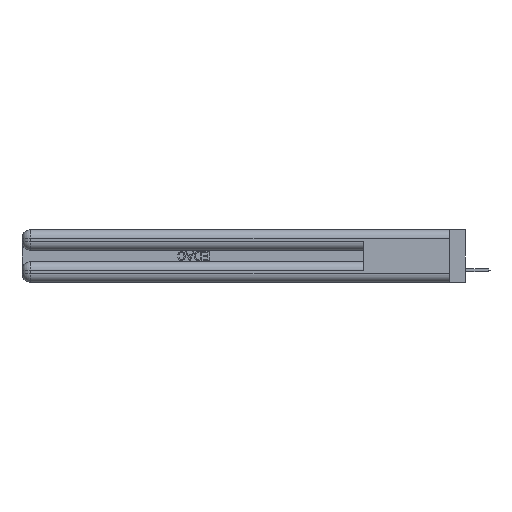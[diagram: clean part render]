
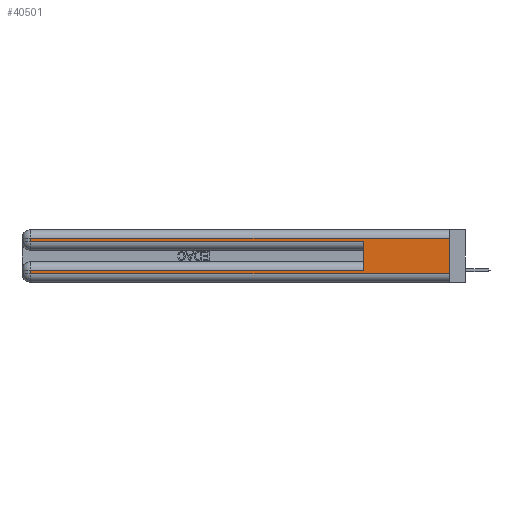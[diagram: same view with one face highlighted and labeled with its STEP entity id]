
A CAD part, left-side view. The second image highlights one B-rep face of the part: STEP entity #40501.
In plain terms, the highlighted planar face has unit normal (-1, 0, 0).
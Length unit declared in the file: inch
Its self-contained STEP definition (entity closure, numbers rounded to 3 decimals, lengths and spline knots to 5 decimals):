
#38 = ORIENTED_EDGE ( 'NONE', *, *, #3209, .T. ) ;
#980 = CARTESIAN_POINT ( 'NONE',  ( 0., 2.94, 0.37 ) ) ;
#3001 = DIRECTION ( 'NONE',  ( 1., 0., 0. ) ) ;
#3209 = EDGE_CURVE ( 'NONE', #36364, #26519, #8917, .T. ) ;
#5085 = VERTEX_POINT ( 'NONE', #32328 ) ;
#5512 = LINE ( 'NONE', #980, #37307 ) ;
#7066 = FACE_OUTER_BOUND ( 'NONE', #13758, .T. ) ;
#8419 = LINE ( 'NONE', #53449, #38146 ) ;
#8917 = LINE ( 'NONE', #11844, #48561 ) ;
#9358 = LINE ( 'NONE', #31911, #36074 ) ;
#9400 = VECTOR ( 'NONE', #47219, 39.37008 ) ;
#9889 = CARTESIAN_POINT ( 'NONE',  ( 0., 2.94, 0.31 ) ) ;
#11844 = CARTESIAN_POINT ( 'NONE',  ( 0., 0., 0.31 ) ) ;
#12064 = EDGE_CURVE ( 'NONE', #26519, #24827, #35401, .T. ) ;
#13758 = EDGE_LOOP ( 'NONE', ( #24534, #38, #50159, #14499, #49826, #46130, #17856, #27384 ) ) ;
#14499 = ORIENTED_EDGE ( 'NONE', *, *, #36199, .T. ) ;
#14515 = LINE ( 'NONE', #39742, #15880 ) ;
#15880 = VECTOR ( 'NONE', #31403, 39.37008 ) ;
#16010 = DIRECTION ( 'NONE',  ( 0., 0., -1. ) ) ;
#17319 = CARTESIAN_POINT ( 'NONE',  ( 0., 0., 0.37 ) ) ;
#17576 = VERTEX_POINT ( 'NONE', #41421 ) ;
#17856 = ORIENTED_EDGE ( 'NONE', *, *, #25757, .T. ) ;
#18302 = CARTESIAN_POINT ( 'NONE',  ( 0., 0., 0.37 ) ) ;
#23362 = EDGE_CURVE ( 'NONE', #23392, #32150, #8419, .T. ) ;
#23392 = VERTEX_POINT ( 'NONE', #47126 ) ;
#23675 = LINE ( 'NONE', #18302, #42400 ) ;
#24534 = ORIENTED_EDGE ( 'NONE', *, *, #44513, .F. ) ;
#24827 = VERTEX_POINT ( 'NONE', #48886 ) ;
#25757 = EDGE_CURVE ( 'NONE', #33454, #17576, #5512, .T. ) ;
#26248 = DIRECTION ( 'NONE',  ( 0., 0., 1. ) ) ;
#26257 = CARTESIAN_POINT ( 'NONE',  ( 0., 2.94, 0.085 ) ) ;
#26311 = DIRECTION ( 'NONE',  ( 0., 0., -1. ) ) ;
#26519 = VERTEX_POINT ( 'NONE', #9889 ) ;
#27384 = ORIENTED_EDGE ( 'NONE', *, *, #44716, .T. ) ;
#28302 = DIRECTION ( 'NONE',  ( 0., 1., 0. ) ) ;
#30276 = DIRECTION ( 'NONE',  ( 0., 0., -1. ) ) ;
#30992 = DIRECTION ( 'NONE',  ( 0., -1., 0. ) ) ;
#31403 = DIRECTION ( 'NONE',  ( 0., -1., 0. ) ) ;
#31911 = CARTESIAN_POINT ( 'NONE',  ( 0., 0., 0.285 ) ) ;
#32150 = VERTEX_POINT ( 'NONE', #51541 ) ;
#32328 = CARTESIAN_POINT ( 'NONE',  ( 0., 0., 0.06 ) ) ;
#33033 = LINE ( 'NONE', #44032, #36967 ) ;
#33454 = VERTEX_POINT ( 'NONE', #26257 ) ;
#35401 = LINE ( 'NONE', #48009, #9400 ) ;
#36074 = VECTOR ( 'NONE', #30992, 39.37008 ) ;
#36199 = EDGE_CURVE ( 'NONE', #24827, #32150, #9358, .T. ) ;
#36364 = VERTEX_POINT ( 'NONE', #39438 ) ;
#36967 = VECTOR ( 'NONE', #28302, 39.37008 ) ;
#37307 = VECTOR ( 'NONE', #26311, 39.37008 ) ;
#38146 = VECTOR ( 'NONE', #26248, 39.37008 ) ;
#39438 = CARTESIAN_POINT ( 'NONE',  ( 0., 0., 0.31 ) ) ;
#39742 = CARTESIAN_POINT ( 'NONE',  ( 0., 0., 0.06 ) ) ;
#40501 = ADVANCED_FACE ( 'NONE', ( #7066 ), #44426, .F. ) ;
#41421 = CARTESIAN_POINT ( 'NONE',  ( 0., 2.94, 0.06 ) ) ;
#42400 = VECTOR ( 'NONE', #30276, 39.37008 ) ;
#44032 = CARTESIAN_POINT ( 'NONE',  ( 0., 0., 0.085 ) ) ;
#44426 = PLANE ( 'NONE',  #45431 ) ;
#44513 = EDGE_CURVE ( 'NONE', #36364, #5085, #23675, .T. ) ;
#44716 = EDGE_CURVE ( 'NONE', #17576, #5085, #14515, .T. ) ;
#45431 = AXIS2_PLACEMENT_3D ( 'NONE', #17319, #3001, #16010 ) ;
#46130 = ORIENTED_EDGE ( 'NONE', *, *, #51348, .T. ) ;
#47126 = CARTESIAN_POINT ( 'NONE',  ( 0., 0.6, 0.085 ) ) ;
#47219 = DIRECTION ( 'NONE',  ( 0., 0., -1. ) ) ;
#48009 = CARTESIAN_POINT ( 'NONE',  ( 0., 2.94, 0.37 ) ) ;
#48561 = VECTOR ( 'NONE', #48981, 39.37008 ) ;
#48886 = CARTESIAN_POINT ( 'NONE',  ( 0., 2.94, 0.285 ) ) ;
#48981 = DIRECTION ( 'NONE',  ( 0., 1., 0. ) ) ;
#49826 = ORIENTED_EDGE ( 'NONE', *, *, #23362, .F. ) ;
#50159 = ORIENTED_EDGE ( 'NONE', *, *, #12064, .T. ) ;
#51348 = EDGE_CURVE ( 'NONE', #23392, #33454, #33033, .T. ) ;
#51541 = CARTESIAN_POINT ( 'NONE',  ( 0., 0.6, 0.285 ) ) ;
#53449 = CARTESIAN_POINT ( 'NONE',  ( 0., 0.6, 0.145 ) ) ;
